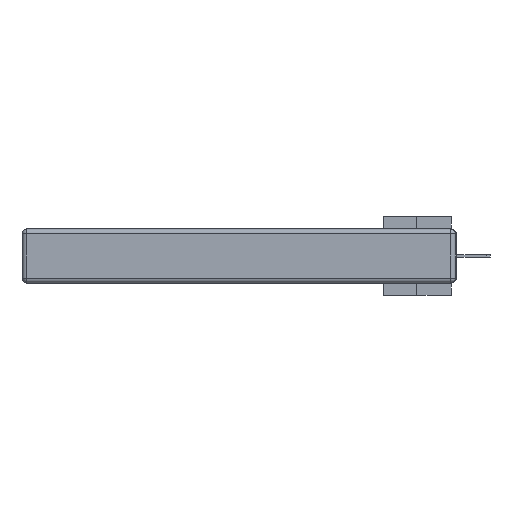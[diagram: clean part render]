
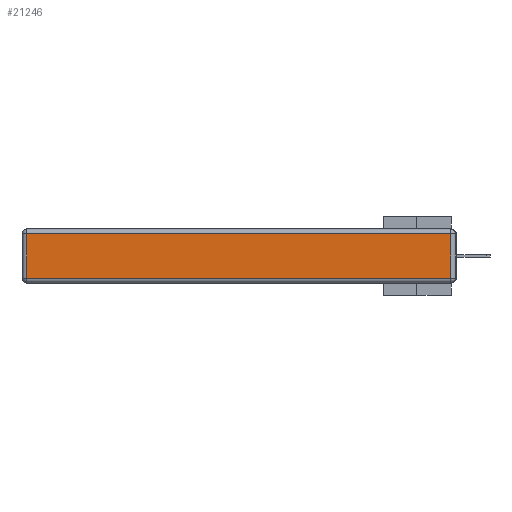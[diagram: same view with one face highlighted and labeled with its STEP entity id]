
A CAD part, left-side view. The second image highlights one B-rep face of the part: STEP entity #21246.
In plain terms, the highlighted planar face has unit normal (-1, 0, 0).
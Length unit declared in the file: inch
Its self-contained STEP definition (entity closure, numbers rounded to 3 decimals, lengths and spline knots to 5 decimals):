
#74 = VECTOR ( 'NONE', #9923, 39.37008 ) ;
#1654 = ORIENTED_EDGE ( 'NONE', *, *, #12002, .T. ) ;
#2074 = DIRECTION ( 'NONE',  ( 0., -1., 0. ) ) ;
#4183 = EDGE_CURVE ( 'NONE', #24254, #28082, #27042, .T. ) ;
#5064 = DIRECTION ( 'NONE',  ( 0., 0., -1. ) ) ;
#5829 = DIRECTION ( 'NONE',  ( 0., 0., 1. ) ) ;
#6658 = LINE ( 'NONE', #29014, #23305 ) ;
#7049 = VECTOR ( 'NONE', #7518, 39.37008 ) ;
#7518 = DIRECTION ( 'NONE',  ( 0., 1., 0. ) ) ;
#7808 = EDGE_CURVE ( 'NONE', #14488, #24254, #20902, .T. ) ;
#9174 = CARTESIAN_POINT ( 'NONE',  ( 0., 0., -0.313 ) ) ;
#9923 = DIRECTION ( 'NONE',  ( 0., 0., 1. ) ) ;
#10494 = EDGE_LOOP ( 'NONE', ( #29453, #10909, #31241, #1654 ) ) ;
#10909 = ORIENTED_EDGE ( 'NONE', *, *, #4183, .T. ) ;
#11203 = LINE ( 'NONE', #29365, #7049 ) ;
#11210 = FACE_OUTER_BOUND ( 'NONE', #10494, .T. ) ;
#11659 = EDGE_CURVE ( 'NONE', #28082, #13804, #11203, .T. ) ;
#12002 = EDGE_CURVE ( 'NONE', #13804, #14488, #6658, .T. ) ;
#12810 = DIRECTION ( 'NONE',  ( -1., 0., 0. ) ) ;
#13031 = CARTESIAN_POINT ( 'NONE',  ( 0., 0., -0.343 ) ) ;
#13804 = VERTEX_POINT ( 'NONE', #28277 ) ;
#14488 = VERTEX_POINT ( 'NONE', #18473 ) ;
#16462 = CARTESIAN_POINT ( 'NONE',  ( 0., 0.03, -0.03 ) ) ;
#18473 = CARTESIAN_POINT ( 'NONE',  ( 0., 2.72, -0.313 ) ) ;
#19919 = PLANE ( 'NONE',  #28809 ) ;
#20667 = CARTESIAN_POINT ( 'NONE',  ( 0., 0.03, -0.313 ) ) ;
#20902 = LINE ( 'NONE', #9174, #25469 ) ;
#21246 = ADVANCED_FACE ( 'NONE', ( #11210 ), #19919, .T. ) ;
#23305 = VECTOR ( 'NONE', #5064, 39.37008 ) ;
#24254 = VERTEX_POINT ( 'NONE', #20667 ) ;
#24465 = CARTESIAN_POINT ( 'NONE',  ( 0., 0.03, -0.343 ) ) ;
#25469 = VECTOR ( 'NONE', #2074, 39.37008 ) ;
#27042 = LINE ( 'NONE', #24465, #74 ) ;
#28082 = VERTEX_POINT ( 'NONE', #16462 ) ;
#28277 = CARTESIAN_POINT ( 'NONE',  ( 0., 2.72, -0.03 ) ) ;
#28809 = AXIS2_PLACEMENT_3D ( 'NONE', #13031, #12810, #5829 ) ;
#29014 = CARTESIAN_POINT ( 'NONE',  ( 0., 2.72, -0.343 ) ) ;
#29365 = CARTESIAN_POINT ( 'NONE',  ( 0., 2.75, -0.03 ) ) ;
#29453 = ORIENTED_EDGE ( 'NONE', *, *, #7808, .T. ) ;
#31241 = ORIENTED_EDGE ( 'NONE', *, *, #11659, .T. ) ;
